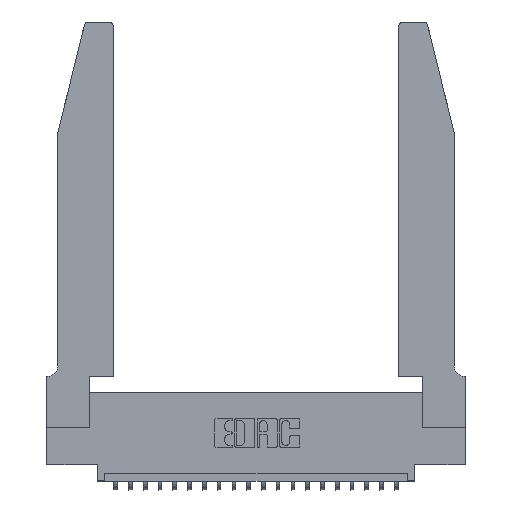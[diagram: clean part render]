
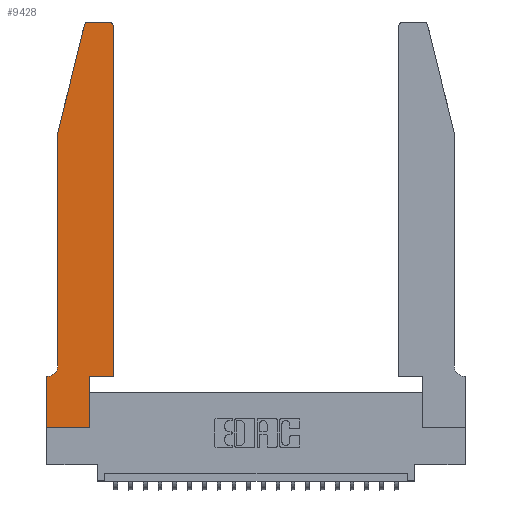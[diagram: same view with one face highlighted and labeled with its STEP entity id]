
A CAD part, top view. The second image highlights one B-rep face of the part: STEP entity #9428.
In plain terms, the highlighted planar face has unit normal (0, 0, 1).
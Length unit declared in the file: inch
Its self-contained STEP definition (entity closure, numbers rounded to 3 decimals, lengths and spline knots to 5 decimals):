
#242 = LINE ( 'NONE', #8973, #10266 ) ;
#551 = DIRECTION ( 'NONE',  ( 1., 0., 0. ) ) ;
#618 = CARTESIAN_POINT ( 'NONE',  ( 0.4505, 0.35, 0.37 ) ) ;
#694 = CARTESIAN_POINT ( 'NONE',  ( 0.0755, 2., 0.37 ) ) ;
#737 = VECTOR ( 'NONE', #22325, 39.37008 ) ;
#1178 = EDGE_CURVE ( 'NONE', #4977, #10152, #12266, .T. ) ;
#1202 = CARTESIAN_POINT ( 'NONE',  ( 0.0055, 0.35, 0.37 ) ) ;
#1301 = DIRECTION ( 'NONE',  ( 0., 0., 1. ) ) ;
#1418 = ORIENTED_EDGE ( 'NONE', *, *, #8687, .T. ) ;
#1607 = VERTEX_POINT ( 'NONE', #1202 ) ;
#2575 = VERTEX_POINT ( 'NONE', #16758 ) ;
#3219 = EDGE_CURVE ( 'NONE', #13126, #10699, #14539, .T. ) ;
#3260 = ORIENTED_EDGE ( 'NONE', *, *, #4220, .T. ) ;
#3293 = DIRECTION ( 'NONE',  ( 0., 1., 0. ) ) ;
#3522 = VERTEX_POINT ( 'NONE', #18688 ) ;
#3531 = ORIENTED_EDGE ( 'NONE', *, *, #5569, .T. ) ;
#4220 = EDGE_CURVE ( 'NONE', #7754, #22382, #10098, .T. ) ;
#4472 = ORIENTED_EDGE ( 'NONE', *, *, #19629, .T. ) ;
#4530 = ORIENTED_EDGE ( 'NONE', *, *, #3219, .T. ) ;
#4895 = LINE ( 'NONE', #694, #16796 ) ;
#4977 = VERTEX_POINT ( 'NONE', #22045 ) ;
#5080 = VECTOR ( 'NONE', #12819, 39.37008 ) ;
#5233 = CIRCLE ( 'NONE', #22103, 0.07 ) ;
#5381 = VECTOR ( 'NONE', #20433, 39.37008 ) ;
#5569 = EDGE_CURVE ( 'NONE', #2575, #4977, #17525, .T. ) ;
#5758 = VERTEX_POINT ( 'NONE', #15965 ) ;
#6008 = CARTESIAN_POINT ( 'NONE',  ( 0.0055, 0.42, 0.37 ) ) ;
#6364 = CARTESIAN_POINT ( 'NONE',  ( 0.284, 2.72, 0.37 ) ) ;
#6486 = EDGE_LOOP ( 'NONE', ( #3531, #19293, #4472, #3260, #20733, #1418, #4530, #16498, #17991, #7192, #21809, #16110 ) ) ;
#6758 = CARTESIAN_POINT ( 'NONE',  ( 0., 0.35, 0.37 ) ) ;
#7192 = ORIENTED_EDGE ( 'NONE', *, *, #11111, .T. ) ;
#7390 = VECTOR ( 'NONE', #9346, 39.37008 ) ;
#7515 = DIRECTION ( 'NONE',  ( 1., 0., 0. ) ) ;
#7754 = VERTEX_POINT ( 'NONE', #18757 ) ;
#7820 = AXIS2_PLACEMENT_3D ( 'NONE', #12692, #10995, #551 ) ;
#7858 = AXIS2_PLACEMENT_3D ( 'NONE', #19011, #1301, #22317 ) ;
#8545 = CARTESIAN_POINT ( 'NONE',  ( 0.2865, 0.35, 0.37 ) ) ;
#8687 = EDGE_CURVE ( 'NONE', #1607, #13126, #16234, .T. ) ;
#8973 = CARTESIAN_POINT ( 'NONE',  ( 0., 0., 0.37 ) ) ;
#9077 = VERTEX_POINT ( 'NONE', #17245 ) ;
#9346 = DIRECTION ( 'NONE',  ( 1., 0., 0. ) ) ;
#9428 = ADVANCED_FACE ( 'NONE', ( #18021 ), #17276, .T. ) ;
#9514 = LINE ( 'NONE', #618, #5080 ) ;
#9532 = CARTESIAN_POINT ( 'NONE',  ( 0.0755, 0.35, 0.37 ) ) ;
#9760 = VECTOR ( 'NONE', #21344, 39.37008 ) ;
#9999 = CARTESIAN_POINT ( 'NONE',  ( 0., 0., 0.37 ) ) ;
#10098 = LINE ( 'NONE', #18947, #5381 ) ;
#10152 = VERTEX_POINT ( 'NONE', #15152 ) ;
#10266 = VECTOR ( 'NONE', #7515, 39.37008 ) ;
#10699 = VERTEX_POINT ( 'NONE', #9999 ) ;
#10995 = DIRECTION ( 'NONE',  ( 0., 0., 1. ) ) ;
#11111 = EDGE_CURVE ( 'NONE', #18874, #5758, #20483, .T. ) ;
#11138 = DIRECTION ( 'NONE',  ( -0.239, -0.971, 0. ) ) ;
#11233 = DIRECTION ( 'NONE',  ( 0., -1., 0. ) ) ;
#11325 = DIRECTION ( 'NONE',  ( -1., 0., 0. ) ) ;
#11636 = LINE ( 'NONE', #8545, #15786 ) ;
#11675 = DIRECTION ( 'NONE',  ( 1., 0., 0. ) ) ;
#11678 = AXIS2_PLACEMENT_3D ( 'NONE', #6364, #18782, #11675 ) ;
#11760 = CARTESIAN_POINT ( 'NONE',  ( 0.0755, 0.42, 0.37 ) ) ;
#12266 = CIRCLE ( 'NONE', #11678, 0.03 ) ;
#12465 = CARTESIAN_POINT ( 'NONE',  ( 0.2605, 2.75, 0.37 ) ) ;
#12692 = CARTESIAN_POINT ( 'NONE',  ( 0.4205, 2.72, 0.37 ) ) ;
#12819 = DIRECTION ( 'NONE',  ( 0., 1., 0. ) ) ;
#13126 = VERTEX_POINT ( 'NONE', #6758 ) ;
#13252 = CIRCLE ( 'NONE', #7820, 0.03 ) ;
#14058 = EDGE_CURVE ( 'NONE', #5758, #3522, #9514, .T. ) ;
#14539 = LINE ( 'NONE', #21866, #20697 ) ;
#14651 = CARTESIAN_POINT ( 'NONE',  ( 0.2865, 0.35, 0.37 ) ) ;
#15152 = CARTESIAN_POINT ( 'NONE',  ( 0.25487, 2.72718, 0.37 ) ) ;
#15786 = VECTOR ( 'NONE', #3293, 39.37008 ) ;
#15934 = EDGE_CURVE ( 'NONE', #9077, #18874, #11636, .T. ) ;
#15965 = CARTESIAN_POINT ( 'NONE',  ( 0.4505, 0.35, 0.37 ) ) ;
#16110 = ORIENTED_EDGE ( 'NONE', *, *, #17314, .T. ) ;
#16234 = LINE ( 'NONE', #9532, #737 ) ;
#16380 = EDGE_CURVE ( 'NONE', #10699, #9077, #242, .T. ) ;
#16498 = ORIENTED_EDGE ( 'NONE', *, *, #16380, .T. ) ;
#16758 = CARTESIAN_POINT ( 'NONE',  ( 0.4205, 2.75, 0.37 ) ) ;
#16796 = VECTOR ( 'NONE', #11138, 39.37008 ) ;
#17239 = EDGE_CURVE ( 'NONE', #22382, #1607, #5233, .T. ) ;
#17245 = CARTESIAN_POINT ( 'NONE',  ( 0.2865, 0., 0.37 ) ) ;
#17276 = PLANE ( 'NONE',  #7858 ) ;
#17314 = EDGE_CURVE ( 'NONE', #3522, #2575, #13252, .T. ) ;
#17525 = LINE ( 'NONE', #12465, #9760 ) ;
#17991 = ORIENTED_EDGE ( 'NONE', *, *, #15934, .T. ) ;
#18021 = FACE_OUTER_BOUND ( 'NONE', #6486, .T. ) ;
#18162 = CARTESIAN_POINT ( 'NONE',  ( 0.4505, 0.35, 0.37 ) ) ;
#18688 = CARTESIAN_POINT ( 'NONE',  ( 0.4505, 2.72, 0.37 ) ) ;
#18757 = CARTESIAN_POINT ( 'NONE',  ( 0.0755, 2., 0.37 ) ) ;
#18782 = DIRECTION ( 'NONE',  ( 0., 0., 1. ) ) ;
#18874 = VERTEX_POINT ( 'NONE', #14651 ) ;
#18947 = CARTESIAN_POINT ( 'NONE',  ( 0.0755, 2., 0.37 ) ) ;
#19011 = CARTESIAN_POINT ( 'NONE',  ( 0., 0.35, 0.37 ) ) ;
#19293 = ORIENTED_EDGE ( 'NONE', *, *, #1178, .T. ) ;
#19629 = EDGE_CURVE ( 'NONE', #10152, #7754, #4895, .T. ) ;
#20210 = DIRECTION ( 'NONE',  ( 0., 0., -1. ) ) ;
#20433 = DIRECTION ( 'NONE',  ( 0., -1., 0. ) ) ;
#20483 = LINE ( 'NONE', #18162, #7390 ) ;
#20697 = VECTOR ( 'NONE', #11233, 39.37008 ) ;
#20733 = ORIENTED_EDGE ( 'NONE', *, *, #17239, .T. ) ;
#21344 = DIRECTION ( 'NONE',  ( -1., 0., 0. ) ) ;
#21809 = ORIENTED_EDGE ( 'NONE', *, *, #14058, .T. ) ;
#21866 = CARTESIAN_POINT ( 'NONE',  ( 0., 0., 0.37 ) ) ;
#22045 = CARTESIAN_POINT ( 'NONE',  ( 0.284, 2.75, 0.37 ) ) ;
#22103 = AXIS2_PLACEMENT_3D ( 'NONE', #6008, #20210, #11325 ) ;
#22317 = DIRECTION ( 'NONE',  ( 1., 0., 0. ) ) ;
#22325 = DIRECTION ( 'NONE',  ( -1., 0., 0. ) ) ;
#22382 = VERTEX_POINT ( 'NONE', #11760 ) ;
